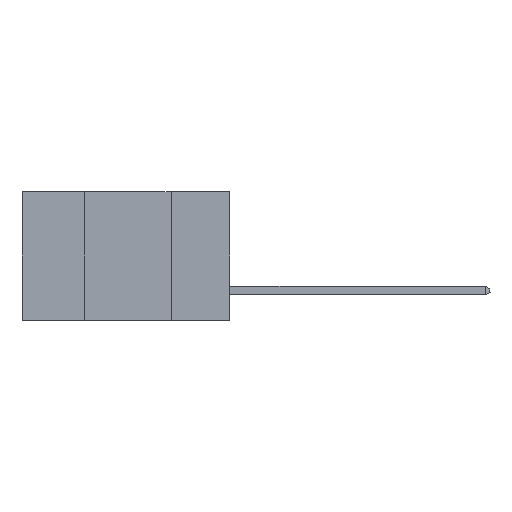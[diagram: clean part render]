
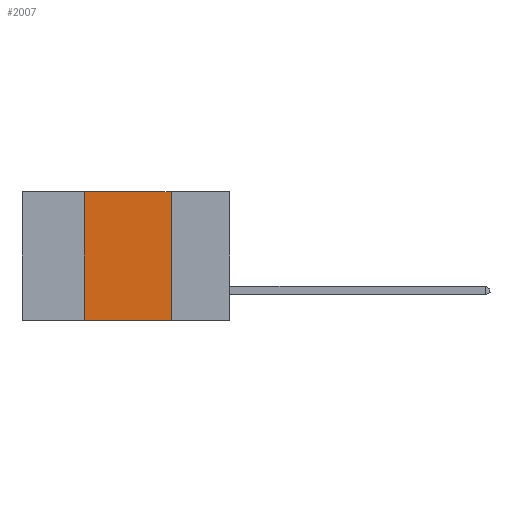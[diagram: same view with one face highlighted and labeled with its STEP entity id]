
A CAD part, left-side view. The second image highlights one B-rep face of the part: STEP entity #2007.
In plain terms, the highlighted planar face has unit normal (-1, 0, 0).
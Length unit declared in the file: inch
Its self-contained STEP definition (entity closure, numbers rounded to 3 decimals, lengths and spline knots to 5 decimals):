
#87 = EDGE_CURVE ( 'NONE', #10185, #3776, #8066, .T. ) ;
#827 = CARTESIAN_POINT ( 'NONE',  ( 0., 0.17, 0. ) ) ;
#1429 = EDGE_LOOP ( 'NONE', ( #8182, #3217, #5525, #6071 ) ) ;
#2007 = ADVANCED_FACE ( 'NONE', ( #11238 ), #8622, .F. ) ;
#2237 = VECTOR ( 'NONE', #6695, 39.37008 ) ;
#2858 = CARTESIAN_POINT ( 'NONE',  ( 0., 0.6, -0.37 ) ) ;
#3085 = EDGE_CURVE ( 'NONE', #9517, #10185, #7584, .T. ) ;
#3217 = ORIENTED_EDGE ( 'NONE', *, *, #87, .F. ) ;
#3420 = CARTESIAN_POINT ( 'NONE',  ( 0., 0.42, 0. ) ) ;
#3776 = VERTEX_POINT ( 'NONE', #827 ) ;
#3940 = LINE ( 'NONE', #3960, #6315 ) ;
#3960 = CARTESIAN_POINT ( 'NONE',  ( 0., 0.17, 0. ) ) ;
#4455 = LINE ( 'NONE', #2858, #2237 ) ;
#4936 = DIRECTION ( 'NONE',  ( 0., -1., 0. ) ) ;
#4995 = CARTESIAN_POINT ( 'NONE',  ( 0., 0.6, 0. ) ) ;
#5007 = CARTESIAN_POINT ( 'NONE',  ( 0., 0.42, 0. ) ) ;
#5525 = ORIENTED_EDGE ( 'NONE', *, *, #3085, .F. ) ;
#5764 = DIRECTION ( 'NONE',  ( 0., 0., -1. ) ) ;
#5919 = DIRECTION ( 'NONE',  ( 1., 0., 0. ) ) ;
#6071 = ORIENTED_EDGE ( 'NONE', *, *, #11351, .T. ) ;
#6315 = VECTOR ( 'NONE', #8611, 39.37008 ) ;
#6436 = AXIS2_PLACEMENT_3D ( 'NONE', #4995, #5919, #5764 ) ;
#6496 = VECTOR ( 'NONE', #4936, 39.37008 ) ;
#6695 = DIRECTION ( 'NONE',  ( 0., -1., 0. ) ) ;
#7584 = LINE ( 'NONE', #5007, #8136 ) ;
#8066 = LINE ( 'NONE', #9707, #6496 ) ;
#8136 = VECTOR ( 'NONE', #9694, 39.37008 ) ;
#8182 = ORIENTED_EDGE ( 'NONE', *, *, #8633, .F. ) ;
#8611 = DIRECTION ( 'NONE',  ( 0., 0., -1. ) ) ;
#8622 = PLANE ( 'NONE',  #6436 ) ;
#8633 = EDGE_CURVE ( 'NONE', #3776, #9169, #3940, .T. ) ;
#9093 = CARTESIAN_POINT ( 'NONE',  ( 0., 0.42, -0.37 ) ) ;
#9169 = VERTEX_POINT ( 'NONE', #10778 ) ;
#9517 = VERTEX_POINT ( 'NONE', #9093 ) ;
#9694 = DIRECTION ( 'NONE',  ( 0., 0., 1. ) ) ;
#9707 = CARTESIAN_POINT ( 'NONE',  ( 0., 0.6, 0. ) ) ;
#10185 = VERTEX_POINT ( 'NONE', #3420 ) ;
#10778 = CARTESIAN_POINT ( 'NONE',  ( 0., 0.17, -0.37 ) ) ;
#11238 = FACE_OUTER_BOUND ( 'NONE', #1429, .T. ) ;
#11351 = EDGE_CURVE ( 'NONE', #9517, #9169, #4455, .T. ) ;
